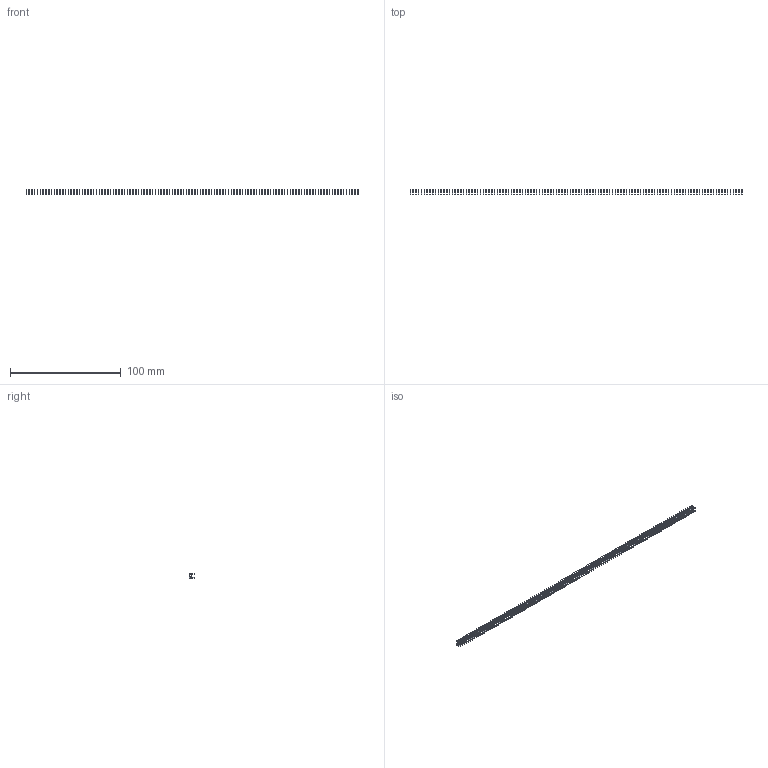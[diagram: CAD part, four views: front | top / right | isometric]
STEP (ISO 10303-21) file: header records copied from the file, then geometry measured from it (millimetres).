
FILE_DESCRIPTION (( 'STEP AP203' ), '1' );
FILE_NAME ('105-119-208-100.STEP', '2020-04-08T01:27:12', ( '' ), ( '' ), 'SwSTEP 2.0', 'SolidWorks 2016', '' );
FILE_SCHEMA (( 'CONFIG_CONTROL_DESIGN' ));
Length unit declared in the file: inch
Products named in the file (2): 100-290-001_100-290-208; 105-119-208-100
Assembly tree (119 placements, depth 2):
  105-119-208-100
    100-290-001_100-290-208  x119
Bounding box: 300.23 x 4.83 x 5.17 mm (x, y, z)
Volume: 818.8 mm3; surface area: 5057 mm2
Topology: 119 solids, 119 shells, 2975 faces, 8211 edges, 5474 vertices
Faces by surface type: plane 2618, cylinder 357
Entity records: 4765 total; most frequent: DIRECTION 369, CARTESIAN_POINT 262, LOCAL_TIME 248, CALENDAR_DATE 248, DATE_AND_TIME 248, COORDINATED_UNIVERSAL_TIME_OFFSET 248, AXIS2_PLACEMENT_3D 153, ORIENTED_EDGE 138
